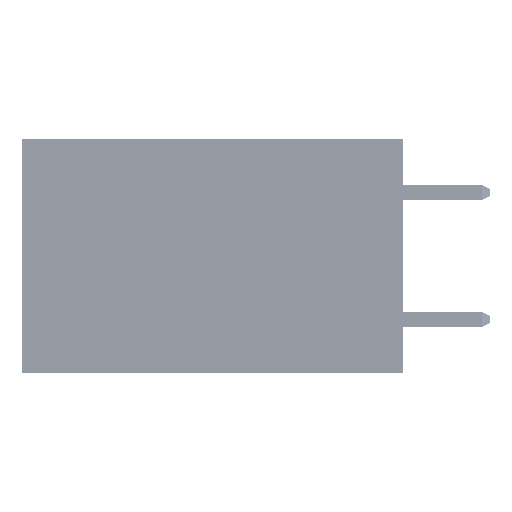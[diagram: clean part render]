
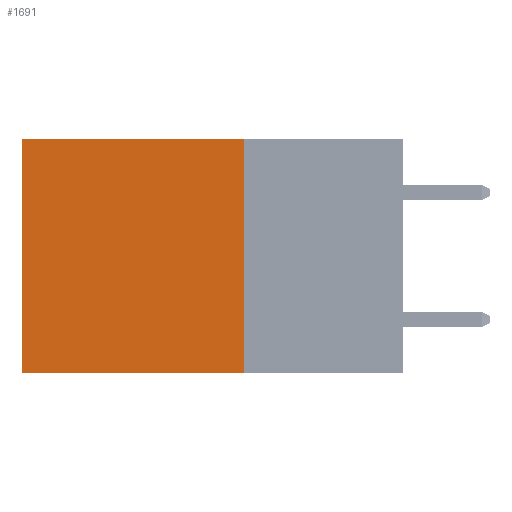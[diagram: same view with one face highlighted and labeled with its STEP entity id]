
A CAD part, left-side view. The second image highlights one B-rep face of the part: STEP entity #1691.
In plain terms, the highlighted planar face has unit normal (-1, 0, 0).
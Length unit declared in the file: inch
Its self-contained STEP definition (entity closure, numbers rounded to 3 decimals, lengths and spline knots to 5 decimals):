
#859 = CARTESIAN_POINT ( 'NONE',  ( 0.2875, 0.25, 0. ) ) ;
#1170 = VERTEX_POINT ( 'NONE', #7482 ) ;
#1403 = VECTOR ( 'NONE', #34054, 39.37008 ) ;
#1691 = ADVANCED_FACE ( 'NONE', ( #16163 ), #30958, .F. ) ;
#2349 = VECTOR ( 'NONE', #2604, 39.37008 ) ;
#2604 = DIRECTION ( 'NONE',  ( 0., 1., 0. ) ) ;
#2707 = EDGE_CURVE ( 'NONE', #11879, #45557, #10192, .T. ) ;
#3073 = CARTESIAN_POINT ( 'NONE',  ( 0.2875, 0.25, 0. ) ) ;
#4935 = DIRECTION ( 'NONE',  ( 1., 0., 0. ) ) ;
#5025 = VERTEX_POINT ( 'NONE', #40017 ) ;
#5077 = VECTOR ( 'NONE', #14264, 39.37008 ) ;
#7482 = CARTESIAN_POINT ( 'NONE',  ( 0.2875, 0.6, 0. ) ) ;
#10128 = EDGE_CURVE ( 'NONE', #11879, #1170, #29843, .T. ) ;
#10192 = LINE ( 'NONE', #859, #1403 ) ;
#11879 = VERTEX_POINT ( 'NONE', #47336 ) ;
#12147 = ORIENTED_EDGE ( 'NONE', *, *, #24191, .F. ) ;
#12844 = CARTESIAN_POINT ( 'NONE',  ( 0.2875, 0.6, 0. ) ) ;
#14264 = DIRECTION ( 'NONE',  ( 0., 1., 0. ) ) ;
#15046 = LINE ( 'NONE', #48099, #5077 ) ;
#16163 = FACE_OUTER_BOUND ( 'NONE', #47197, .T. ) ;
#20722 = ORIENTED_EDGE ( 'NONE', *, *, #36309, .T. ) ;
#22189 = ORIENTED_EDGE ( 'NONE', *, *, #2707, .F. ) ;
#24191 = EDGE_CURVE ( 'NONE', #45557, #5025, #15046, .T. ) ;
#25653 = CARTESIAN_POINT ( 'NONE',  ( 0.2875, 0.25, -0.37 ) ) ;
#26981 = DIRECTION ( 'NONE',  ( 0., 0., -1. ) ) ;
#28037 = CARTESIAN_POINT ( 'NONE',  ( 0.2875, 0.25, 0. ) ) ;
#28217 = LINE ( 'NONE', #12844, #36377 ) ;
#29843 = LINE ( 'NONE', #3073, #2349 ) ;
#30958 = PLANE ( 'NONE',  #43943 ) ;
#31163 = ORIENTED_EDGE ( 'NONE', *, *, #10128, .T. ) ;
#34054 = DIRECTION ( 'NONE',  ( 0., 0., -1. ) ) ;
#36309 = EDGE_CURVE ( 'NONE', #1170, #5025, #28217, .T. ) ;
#36377 = VECTOR ( 'NONE', #46634, 39.37008 ) ;
#40017 = CARTESIAN_POINT ( 'NONE',  ( 0.2875, 0.6, -0.37 ) ) ;
#43943 = AXIS2_PLACEMENT_3D ( 'NONE', #28037, #4935, #26981 ) ;
#45557 = VERTEX_POINT ( 'NONE', #25653 ) ;
#46634 = DIRECTION ( 'NONE',  ( 0., 0., -1. ) ) ;
#47197 = EDGE_LOOP ( 'NONE', ( #20722, #12147, #22189, #31163 ) ) ;
#47336 = CARTESIAN_POINT ( 'NONE',  ( 0.2875, 0.25, 0. ) ) ;
#48099 = CARTESIAN_POINT ( 'NONE',  ( 0.2875, 0.25, -0.37 ) ) ;
